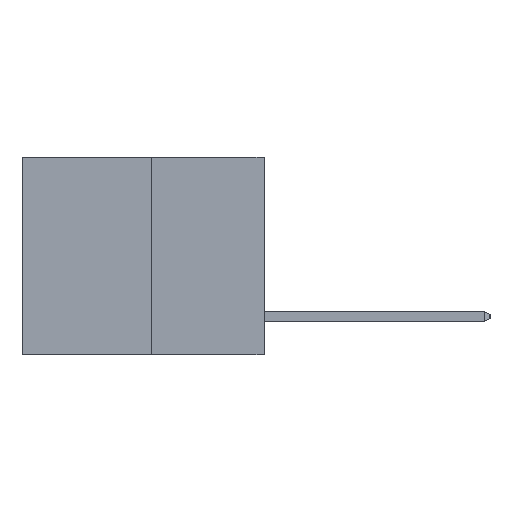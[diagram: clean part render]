
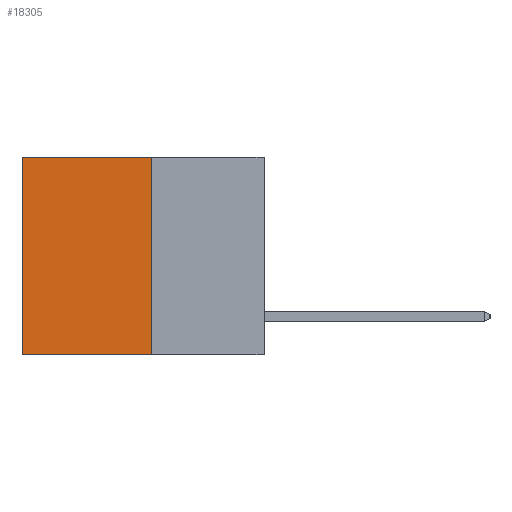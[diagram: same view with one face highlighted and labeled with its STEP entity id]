
A CAD part, left-side view. The second image highlights one B-rep face of the part: STEP entity #18305.
In plain terms, the highlighted planar face has unit normal (-1, 0, 0).
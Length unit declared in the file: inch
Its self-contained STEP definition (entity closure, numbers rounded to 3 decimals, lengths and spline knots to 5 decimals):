
#343 = DIRECTION ( 'NONE',  ( 1., 0., 0. ) ) ;
#1667 = EDGE_CURVE ( 'NONE', #14611, #21447, #22323, .T. ) ;
#2148 = CARTESIAN_POINT ( 'NONE',  ( 0.3165, 0.28, 0. ) ) ;
#4464 = DIRECTION ( 'NONE',  ( 0., 1., 0. ) ) ;
#4512 = VERTEX_POINT ( 'NONE', #10206 ) ;
#4555 = CARTESIAN_POINT ( 'NONE',  ( 0.3165, 0.28, -0.49 ) ) ;
#4700 = VECTOR ( 'NONE', #20497, 39.37008 ) ;
#5409 = PLANE ( 'NONE',  #13535 ) ;
#7253 = LINE ( 'NONE', #2148, #7617 ) ;
#7497 = CARTESIAN_POINT ( 'NONE',  ( 0.3165, 0.6, -0.49 ) ) ;
#7617 = VECTOR ( 'NONE', #13974, 39.37008 ) ;
#8323 = LINE ( 'NONE', #4555, #4700 ) ;
#9038 = CARTESIAN_POINT ( 'NONE',  ( 0.3165, 0.28, -0.49 ) ) ;
#9619 = DIRECTION ( 'NONE',  ( 0., 0., -1. ) ) ;
#9983 = VERTEX_POINT ( 'NONE', #19249 ) ;
#10206 = CARTESIAN_POINT ( 'NONE',  ( 0.3165, 0.28, 0. ) ) ;
#10257 = ORIENTED_EDGE ( 'NONE', *, *, #21690, .F. ) ;
#11008 = LINE ( 'NONE', #7497, #28397 ) ;
#12062 = FACE_OUTER_BOUND ( 'NONE', #14814, .T. ) ;
#12203 = DIRECTION ( 'NONE',  ( 0., 0., -1. ) ) ;
#13535 = AXIS2_PLACEMENT_3D ( 'NONE', #21346, #343, #9619 ) ;
#13974 = DIRECTION ( 'NONE',  ( 0., 1., 0. ) ) ;
#14611 = VERTEX_POINT ( 'NONE', #9038 ) ;
#14814 = EDGE_LOOP ( 'NONE', ( #24345, #26521, #10257, #24821 ) ) ;
#15052 = CARTESIAN_POINT ( 'NONE',  ( 0.3165, 0.6, -0.49 ) ) ;
#18305 = ADVANCED_FACE ( 'NONE', ( #12062 ), #5409, .F. ) ;
#19249 = CARTESIAN_POINT ( 'NONE',  ( 0.3165, 0.6, 0. ) ) ;
#19516 = EDGE_CURVE ( 'NONE', #9983, #21447, #11008, .T. ) ;
#20497 = DIRECTION ( 'NONE',  ( 0., 0., -1. ) ) ;
#21085 = EDGE_CURVE ( 'NONE', #4512, #9983, #7253, .T. ) ;
#21346 = CARTESIAN_POINT ( 'NONE',  ( 0.3165, 0.28, -0.49 ) ) ;
#21447 = VERTEX_POINT ( 'NONE', #15052 ) ;
#21572 = VECTOR ( 'NONE', #4464, 39.37008 ) ;
#21690 = EDGE_CURVE ( 'NONE', #4512, #14611, #8323, .T. ) ;
#22323 = LINE ( 'NONE', #29362, #21572 ) ;
#24345 = ORIENTED_EDGE ( 'NONE', *, *, #19516, .T. ) ;
#24821 = ORIENTED_EDGE ( 'NONE', *, *, #21085, .T. ) ;
#26521 = ORIENTED_EDGE ( 'NONE', *, *, #1667, .F. ) ;
#28397 = VECTOR ( 'NONE', #12203, 39.37008 ) ;
#29362 = CARTESIAN_POINT ( 'NONE',  ( 0.3165, 0.28, -0.49 ) ) ;
